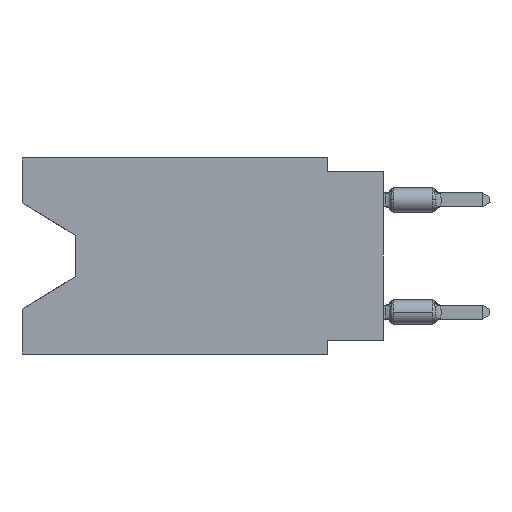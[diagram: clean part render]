
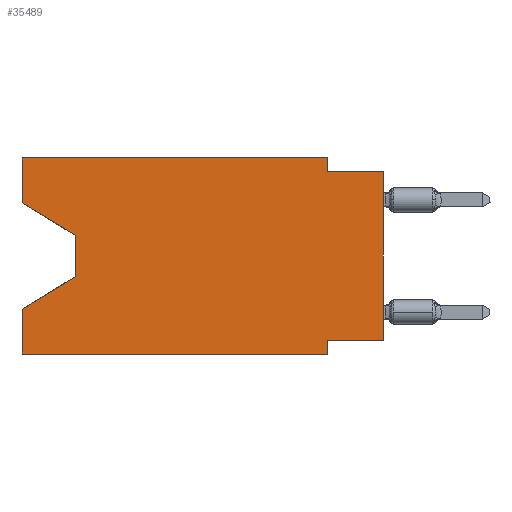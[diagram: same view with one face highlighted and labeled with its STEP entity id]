
A CAD part, left-side view. The second image highlights one B-rep face of the part: STEP entity #35489.
In plain terms, the highlighted planar face has unit normal (-1, 0, 0).
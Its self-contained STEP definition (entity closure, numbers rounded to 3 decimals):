
#215 = CARTESIAN_POINT ( 'NONE',  ( 0., 16.383, -8.89 ) ) ;
#1233 = LINE ( 'NONE', #7210, #32273 ) ;
#1776 = VECTOR ( 'NONE', #15084, 1000. ) ;
#2522 = CARTESIAN_POINT ( 'NONE',  ( 0., 2.54, -8.89 ) ) ;
#2685 = VECTOR ( 'NONE', #21164, 1000. ) ;
#3127 = DIRECTION ( 'NONE',  ( 0., -1., 0. ) ) ;
#3696 = EDGE_CURVE ( 'NONE', #35249, #34906, #8733, .T. ) ;
#3763 = ORIENTED_EDGE ( 'NONE', *, *, #3696, .T. ) ;
#3803 = FACE_OUTER_BOUND ( 'NONE', #35813, .T. ) ;
#4107 = EDGE_CURVE ( 'NONE', #6137, #38176, #15882, .T. ) ;
#4347 = EDGE_CURVE ( 'NONE', #40567, #20509, #22896, .T. ) ;
#4468 = CARTESIAN_POINT ( 'NONE',  ( 0., 13.97, -3.505 ) ) ;
#4592 = VECTOR ( 'NONE', #27145, 1000. ) ;
#4780 = EDGE_CURVE ( 'NONE', #20031, #32570, #38523, .T. ) ;
#5034 = ORIENTED_EDGE ( 'NONE', *, *, #4780, .F. ) ;
#6137 = VERTEX_POINT ( 'NONE', #33232 ) ;
#6867 = EDGE_CURVE ( 'NONE', #22304, #18900, #39720, .T. ) ;
#7023 = LINE ( 'NONE', #215, #18530 ) ;
#7188 = DIRECTION ( 'NONE',  ( 0., 0., -1. ) ) ;
#7210 = CARTESIAN_POINT ( 'NONE',  ( 0., 16.383, 0. ) ) ;
#7377 = VECTOR ( 'NONE', #33838, 1000. ) ;
#7558 = CARTESIAN_POINT ( 'NONE',  ( 0., 13.97, -3.505 ) ) ;
#8733 = LINE ( 'NONE', #33924, #32899 ) ;
#8839 = DIRECTION ( 'NONE',  ( 0., 1., 0. ) ) ;
#8843 = CARTESIAN_POINT ( 'NONE',  ( 0., 0., -0.635 ) ) ;
#9008 = CARTESIAN_POINT ( 'NONE',  ( 0., 13.97, -5.385 ) ) ;
#9376 = CARTESIAN_POINT ( 'NONE',  ( 0., 2.54, 0. ) ) ;
#9857 = CARTESIAN_POINT ( 'NONE',  ( 0., 16.383, -2.038 ) ) ;
#10622 = VECTOR ( 'NONE', #30077, 1000. ) ;
#11272 = VERTEX_POINT ( 'NONE', #23602 ) ;
#12344 = LINE ( 'NONE', #8843, #7377 ) ;
#14566 = CARTESIAN_POINT ( 'NONE',  ( 0., 16.383, 0. ) ) ;
#15084 = DIRECTION ( 'NONE',  ( 0., 0., 1. ) ) ;
#15882 = LINE ( 'NONE', #9857, #24991 ) ;
#16396 = DIRECTION ( 'NONE',  ( 1., 0., 0. ) ) ;
#18225 = ORIENTED_EDGE ( 'NONE', *, *, #6867, .T. ) ;
#18523 = EDGE_CURVE ( 'NONE', #6137, #31591, #33863, .T. ) ;
#18530 = VECTOR ( 'NONE', #3127, 1000. ) ;
#18758 = ORIENTED_EDGE ( 'NONE', *, *, #18523, .F. ) ;
#18900 = VERTEX_POINT ( 'NONE', #37189 ) ;
#19269 = ORIENTED_EDGE ( 'NONE', *, *, #4107, .T. ) ;
#19311 = CARTESIAN_POINT ( 'NONE',  ( 0., 0., -8.255 ) ) ;
#20031 = VERTEX_POINT ( 'NONE', #37692 ) ;
#20189 = ORIENTED_EDGE ( 'NONE', *, *, #26060, .F. ) ;
#20509 = VERTEX_POINT ( 'NONE', #22141 ) ;
#21164 = DIRECTION ( 'NONE',  ( 0., -1., 0. ) ) ;
#21478 = EDGE_CURVE ( 'NONE', #11272, #34906, #1233, .T. ) ;
#21905 = ORIENTED_EDGE ( 'NONE', *, *, #4347, .F. ) ;
#22141 = CARTESIAN_POINT ( 'NONE',  ( 0., 2.54, -0.635 ) ) ;
#22202 = ORIENTED_EDGE ( 'NONE', *, *, #38151, .T. ) ;
#22304 = VERTEX_POINT ( 'NONE', #19311 ) ;
#22679 = DIRECTION ( 'NONE',  ( 0., -0.855, -0.519 ) ) ;
#22772 = AXIS2_PLACEMENT_3D ( 'NONE', #22808, #16396, #28979 ) ;
#22808 = CARTESIAN_POINT ( 'NONE',  ( 0., 16.383, 0. ) ) ;
#22896 = LINE ( 'NONE', #36116, #30287 ) ;
#23602 = CARTESIAN_POINT ( 'NONE',  ( 0., 16.383, -8.89 ) ) ;
#24044 = CARTESIAN_POINT ( 'NONE',  ( 0., 0., 0. ) ) ;
#24298 = EDGE_CURVE ( 'NONE', #11272, #32570, #7023, .T. ) ;
#24991 = VECTOR ( 'NONE', #22679, 1000. ) ;
#25157 = CARTESIAN_POINT ( 'NONE',  ( 0., 16.383, -6.852 ) ) ;
#26060 = EDGE_CURVE ( 'NONE', #20509, #18900, #12344, .T. ) ;
#26352 = CARTESIAN_POINT ( 'NONE',  ( 0., 2.54, -8.89 ) ) ;
#27062 = CARTESIAN_POINT ( 'NONE',  ( 0., 16.383, 0. ) ) ;
#27145 = DIRECTION ( 'NONE',  ( 0., 0., -1. ) ) ;
#27817 = ORIENTED_EDGE ( 'NONE', *, *, #40743, .F. ) ;
#28979 = DIRECTION ( 'NONE',  ( 0., 0., -1. ) ) ;
#29423 = ORIENTED_EDGE ( 'NONE', *, *, #33765, .F. ) ;
#30077 = DIRECTION ( 'NONE',  ( 0., 0., -1. ) ) ;
#30287 = VECTOR ( 'NONE', #7188, 1000. ) ;
#31224 = DIRECTION ( 'NONE',  ( 0., 0.855, -0.519 ) ) ;
#31591 = VERTEX_POINT ( 'NONE', #32835 ) ;
#31683 = PLANE ( 'NONE',  #22772 ) ;
#32273 = VECTOR ( 'NONE', #38382, 1000. ) ;
#32570 = VERTEX_POINT ( 'NONE', #2522 ) ;
#32835 = CARTESIAN_POINT ( 'NONE',  ( 0., 16.383, 0. ) ) ;
#32899 = VECTOR ( 'NONE', #31224, 1000. ) ;
#33232 = CARTESIAN_POINT ( 'NONE',  ( 0., 16.383, -2.038 ) ) ;
#33442 = VECTOR ( 'NONE', #36007, 1000. ) ;
#33765 = EDGE_CURVE ( 'NONE', #22304, #20031, #37134, .T. ) ;
#33836 = CARTESIAN_POINT ( 'NONE',  ( 0., 0., -8.255 ) ) ;
#33838 = DIRECTION ( 'NONE',  ( 0., -1., 0. ) ) ;
#33863 = LINE ( 'NONE', #27062, #1776 ) ;
#33924 = CARTESIAN_POINT ( 'NONE',  ( 0., 13.97, -5.385 ) ) ;
#33950 = ORIENTED_EDGE ( 'NONE', *, *, #24298, .T. ) ;
#34345 = ORIENTED_EDGE ( 'NONE', *, *, #21478, .F. ) ;
#34507 = VECTOR ( 'NONE', #8839, 1000. ) ;
#34906 = VERTEX_POINT ( 'NONE', #25157 ) ;
#35249 = VERTEX_POINT ( 'NONE', #9008 ) ;
#35489 = ADVANCED_FACE ( 'NONE', ( #3803 ), #31683, .F. ) ;
#35813 = EDGE_LOOP ( 'NONE', ( #19269, #22202, #3763, #34345, #33950, #5034, #29423, #18225, #20189, #21905, #27817, #18758 ) ) ;
#36007 = DIRECTION ( 'NONE',  ( 0., 0., 1. ) ) ;
#36059 = LINE ( 'NONE', #4468, #10622 ) ;
#36116 = CARTESIAN_POINT ( 'NONE',  ( 0., 2.54, 0. ) ) ;
#37134 = LINE ( 'NONE', #33836, #34507 ) ;
#37189 = CARTESIAN_POINT ( 'NONE',  ( 0., 0., -0.635 ) ) ;
#37692 = CARTESIAN_POINT ( 'NONE',  ( 0., 2.54, -8.255 ) ) ;
#38151 = EDGE_CURVE ( 'NONE', #38176, #35249, #36059, .T. ) ;
#38176 = VERTEX_POINT ( 'NONE', #7558 ) ;
#38382 = DIRECTION ( 'NONE',  ( 0., 0., 1. ) ) ;
#38523 = LINE ( 'NONE', #26352, #4592 ) ;
#39548 = LINE ( 'NONE', #14566, #2685 ) ;
#39720 = LINE ( 'NONE', #24044, #33442 ) ;
#40567 = VERTEX_POINT ( 'NONE', #9376 ) ;
#40743 = EDGE_CURVE ( 'NONE', #31591, #40567, #39548, .T. ) ;
